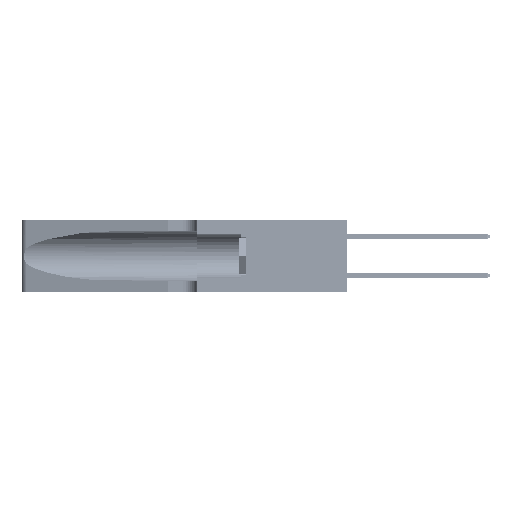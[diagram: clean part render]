
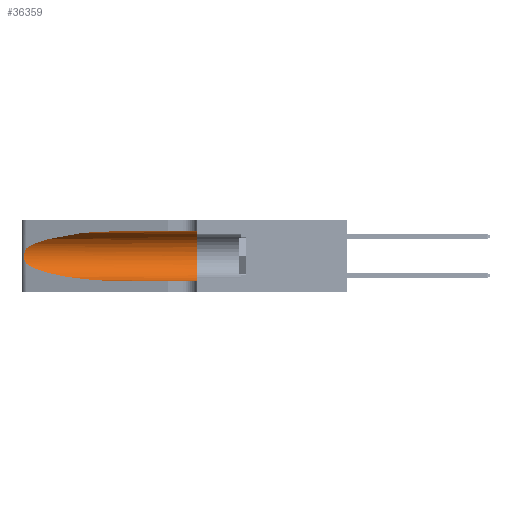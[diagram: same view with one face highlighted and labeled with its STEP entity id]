
A CAD part, left-side view. The second image highlights one B-rep face of the part: STEP entity #36359.
In plain terms, the highlighted cylindrical face has radius 3.308 mm (diameter 6.617 mm), a partial arc.
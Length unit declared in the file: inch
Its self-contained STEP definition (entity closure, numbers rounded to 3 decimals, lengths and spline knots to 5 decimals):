
#815 = CARTESIAN_POINT ( 'NONE',  ( 0.25555, 1.22994, 0.2215 ) ) ;
#1175 = EDGE_CURVE ( 'NONE', #47573, #16083, #32697, .T. ) ;
#2995 = CARTESIAN_POINT ( 'NONE',  ( 0.18966, 0.96281, 0.31525 ) ) ;
#4297 = CARTESIAN_POINT ( 'NONE',  ( 0.25487, 1.22718, 0.22369 ) ) ;
#4604 = ORIENTED_EDGE ( 'NONE', *, *, #14696, .T. ) ;
#6293 = EDGE_CURVE ( 'NONE', #22609, #13819, #54423, .T. ) ;
#6366 = CARTESIAN_POINT ( 'NONE',  ( 0.1305, 0.72297, 0.05475 ) ) ;
#7147 =( BOUNDED_CURVE ( )  B_SPLINE_CURVE ( 3, ( #52586, #31731, #40266, #6366 ),
 .UNSPECIFIED., .F., .F. ) 
 B_SPLINE_CURVE_WITH_KNOTS ( ( 4, 4 ),
 ( 3.44316, 4.71239 ),
 .UNSPECIFIED. ) 
 CURVE ( )  GEOMETRIC_REPRESENTATION_ITEM ( )  RATIONAL_B_SPLINE_CURVE ( ( 1., 0.87, 0.87, 1. ) ) 
 REPRESENTATION_ITEM ( '' )  );
#7789 = CARTESIAN_POINT ( 'NONE',  ( 0.25487, 1.22718, 0.22369 ) ) ;
#8380 = CARTESIAN_POINT ( 'NONE',  ( 0.25787, 1.23484, 0.2124 ) ) ;
#8736 = CARTESIAN_POINT ( 'NONE',  ( 0.25856, 1.23593, 0.16098 ) ) ;
#9095 = CARTESIAN_POINT ( 'NONE',  ( 0.25854, 1.2359, 0.20912 ) ) ;
#13819 = VERTEX_POINT ( 'NONE', #35472 ) ;
#14135 = EDGE_CURVE ( 'NONE', #13819, #25125, #27387, .T. ) ;
#14677 = EDGE_LOOP ( 'NONE', ( #48435, #31041, #54329, #4604, #29332, #18192 ) ) ;
#14696 = EDGE_CURVE ( 'NONE', #16223, #16083, #46403, .T. ) ;
#15366 = CARTESIAN_POINT ( 'NONE',  ( 0.1305, 0.72297, 0.31525 ) ) ;
#16083 = VERTEX_POINT ( 'NONE', #46676 ) ;
#16223 = VERTEX_POINT ( 'NONE', #30441 ) ;
#16874 = CARTESIAN_POINT ( 'NONE',  ( 0.26018, 1.23835, 0.19895 ) ) ;
#17007 = DIRECTION ( 'NONE',  ( 0., -1., 0. ) ) ;
#17412 = CARTESIAN_POINT ( 'NONE',  ( 0.25789, 1.23486, 0.15765 ) ) ;
#17592 = CARTESIAN_POINT ( 'NONE',  ( 0.25487, 1.22718, 0.14631 ) ) ;
#18192 = ORIENTED_EDGE ( 'NONE', *, *, #33614, .F. ) ;
#19647 = CARTESIAN_POINT ( 'NONE',  ( 0.1305, 0.35, 0.31525 ) ) ;
#21130 = CARTESIAN_POINT ( 'NONE',  ( 0.25487, 1.22718, 0.14631 ) ) ;
#21282 = CARTESIAN_POINT ( 'NONE',  ( 0.25555, 1.22993, 0.14849 ) ) ;
#21824 = CARTESIAN_POINT ( 'NONE',  ( 0.25639, 1.23186, 0.15144 ) ) ;
#22609 = VERTEX_POINT ( 'NONE', #26882 ) ;
#25125 = VERTEX_POINT ( 'NONE', #21130 ) ;
#25672 = CARTESIAN_POINT ( 'NONE',  ( 0.26075, 1.23896, 0.19203 ) ) ;
#26882 = CARTESIAN_POINT ( 'NONE',  ( 0.1305, 0.72297, 0.31525 ) ) ;
#26905 = CARTESIAN_POINT ( 'NONE',  ( 0.1305, 1.61858, 0.31525 ) ) ;
#27387 = B_SPLINE_CURVE_WITH_KNOTS ( 'NONE', 3,
 ( #4297, #815, #46667, #8380, #9095, #16874, #25672, #51284, #30069, #8736, #17412, #21824, #21282, #17592 ),
 .UNSPECIFIED., .F., .F.,
 ( 4, 2, 2, 2, 2, 2, 4 ),
 ( 0., 0.00027, 0.00053, 0.00107, 0.0016, 0.00187, 0.00214 ),
 .UNSPECIFIED. ) ;
#29332 = ORIENTED_EDGE ( 'NONE', *, *, #1175, .F. ) ;
#30069 = CARTESIAN_POINT ( 'NONE',  ( 0.26017, 1.23833, 0.17102 ) ) ;
#30441 = CARTESIAN_POINT ( 'NONE',  ( 0.1305, 0.72297, 0.05475 ) ) ;
#31041 = ORIENTED_EDGE ( 'NONE', *, *, #14135, .T. ) ;
#31731 = CARTESIAN_POINT ( 'NONE',  ( 0.2373, 1.15595, 0.08982 ) ) ;
#32269 = CARTESIAN_POINT ( 'NONE',  ( 0.2373, 1.15595, 0.28018 ) ) ;
#32697 = CIRCLE ( 'NONE', #45179, 0.13025 ) ;
#33614 = EDGE_CURVE ( 'NONE', #22609, #47573, #52766, .T. ) ;
#35190 = VECTOR ( 'NONE', #37249, 39.37008 ) ;
#35472 = CARTESIAN_POINT ( 'NONE',  ( 0.25487, 1.22718, 0.22369 ) ) ;
#35541 = DIRECTION ( 'NONE',  ( 0., -1., 0. ) ) ;
#36359 = ADVANCED_FACE ( 'NONE', ( #49314 ), #47296, .F. ) ;
#37249 = DIRECTION ( 'NONE',  ( 0., -1., 0. ) ) ;
#37631 = DIRECTION ( 'NONE',  ( 0., 0., -1. ) ) ;
#38297 = VECTOR ( 'NONE', #35541, 39.37008 ) ;
#40266 = CARTESIAN_POINT ( 'NONE',  ( 0.18966, 0.96281, 0.05475 ) ) ;
#40886 = DIRECTION ( 'NONE',  ( 0., 0., 1. ) ) ;
#45179 = AXIS2_PLACEMENT_3D ( 'NONE', #53204, #49689, #40886 ) ;
#46403 = LINE ( 'NONE', #54378, #35190 ) ;
#46667 = CARTESIAN_POINT ( 'NONE',  ( 0.25639, 1.23184, 0.21858 ) ) ;
#46676 = CARTESIAN_POINT ( 'NONE',  ( 0.1305, 0.35, 0.05475 ) ) ;
#47296 = CYLINDRICAL_SURFACE ( 'NONE', #48064, 0.13025 ) ;
#47573 = VERTEX_POINT ( 'NONE', #19647 ) ;
#48064 = AXIS2_PLACEMENT_3D ( 'NONE', #50524, #17007, #37631 ) ;
#48435 = ORIENTED_EDGE ( 'NONE', *, *, #6293, .T. ) ;
#49314 = FACE_OUTER_BOUND ( 'NONE', #14677, .T. ) ;
#49689 = DIRECTION ( 'NONE',  ( 0., 1., 0. ) ) ;
#50524 = CARTESIAN_POINT ( 'NONE',  ( 0.1305, 1.61858, 0.185 ) ) ;
#51284 = CARTESIAN_POINT ( 'NONE',  ( 0.26075, 1.23896, 0.178 ) ) ;
#52586 = CARTESIAN_POINT ( 'NONE',  ( 0.25487, 1.22718, 0.14631 ) ) ;
#52766 = LINE ( 'NONE', #26905, #38297 ) ;
#53204 = CARTESIAN_POINT ( 'NONE',  ( 0.1305, 0.35, 0.185 ) ) ;
#54153 = EDGE_CURVE ( 'NONE', #25125, #16223, #7147, .T. ) ;
#54329 = ORIENTED_EDGE ( 'NONE', *, *, #54153, .T. ) ;
#54378 = CARTESIAN_POINT ( 'NONE',  ( 0.1305, 1.61858, 0.05475 ) ) ;
#54423 =( BOUNDED_CURVE ( )  B_SPLINE_CURVE ( 3, ( #15366, #2995, #32269, #7789 ),
 .UNSPECIFIED., .F., .T. ) 
 B_SPLINE_CURVE_WITH_KNOTS ( ( 4, 4 ),
 ( 1.5708, 2.84003 ),
 .UNSPECIFIED. ) 
 CURVE ( )  GEOMETRIC_REPRESENTATION_ITEM ( )  RATIONAL_B_SPLINE_CURVE ( ( 1., 0.87, 0.87, 1. ) ) 
 REPRESENTATION_ITEM ( '' )  );
